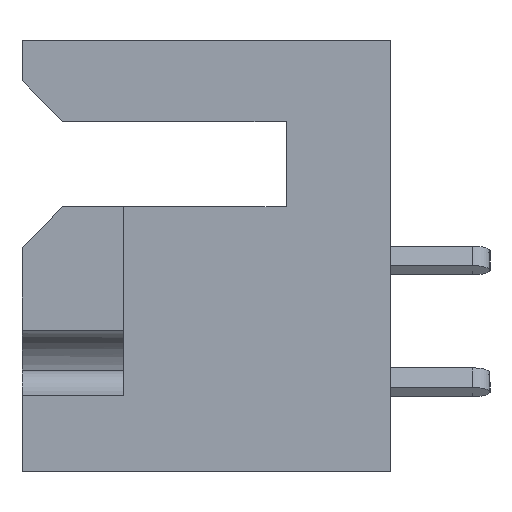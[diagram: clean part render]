
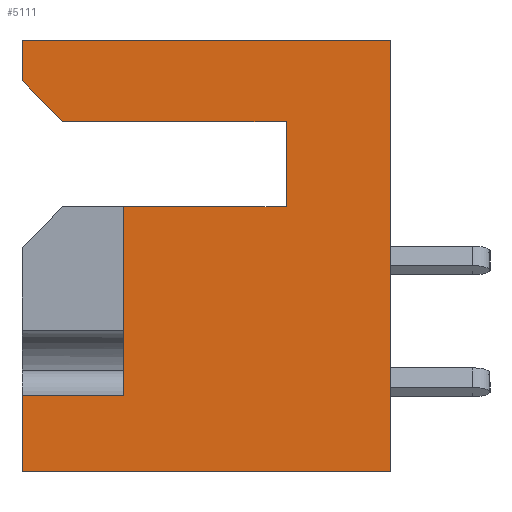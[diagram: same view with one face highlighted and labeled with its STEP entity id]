
A CAD part, left-side view. The second image highlights one B-rep face of the part: STEP entity #5111.
In plain terms, the highlighted planar face has unit normal (-1, 0, 0).
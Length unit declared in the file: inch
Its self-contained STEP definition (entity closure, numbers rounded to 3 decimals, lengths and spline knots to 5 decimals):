
#319 = VECTOR ( 'NONE', #18243, 39.37008 ) ;
#774 = ORIENTED_EDGE ( 'NONE', *, *, #8743, .T. ) ;
#1271 = CARTESIAN_POINT ( 'NONE',  ( 0., 0.453, 0. ) ) ;
#1697 = AXIS2_PLACEMENT_3D ( 'NONE', #1271, #28110, #20865 ) ;
#1863 = CARTESIAN_POINT ( 'NONE',  ( 0., 0.128, -0.1 ) ) ;
#2081 = CARTESIAN_POINT ( 'NONE',  ( 0., 0.453, -0.531 ) ) ;
#2259 = VERTEX_POINT ( 'NONE', #21625 ) ;
#2422 = CARTESIAN_POINT ( 'NONE',  ( 0., 0.328, -0.205 ) ) ;
#3180 = ORIENTED_EDGE ( 'NONE', *, *, #5349, .T. ) ;
#3526 = CARTESIAN_POINT ( 'NONE',  ( 0., 0.403, -0.1 ) ) ;
#3631 = VERTEX_POINT ( 'NONE', #2422 ) ;
#3748 = ORIENTED_EDGE ( 'NONE', *, *, #29592, .T. ) ;
#4726 = LINE ( 'NONE', #18742, #27573 ) ;
#4788 = DIRECTION ( 'NONE',  ( 0., -1., 0. ) ) ;
#5111 = ADVANCED_FACE ( 'NONE', ( #18827 ), #25651, .F. ) ;
#5130 = EDGE_CURVE ( 'NONE', #6974, #15031, #21159, .T. ) ;
#5163 = VERTEX_POINT ( 'NONE', #20975 ) ;
#5301 = VERTEX_POINT ( 'NONE', #15637 ) ;
#5349 = EDGE_CURVE ( 'NONE', #24979, #2259, #16015, .T. ) ;
#6956 = CARTESIAN_POINT ( 'NONE',  ( 0., 0.328, -0.205 ) ) ;
#6965 = LINE ( 'NONE', #28628, #15486 ) ;
#6974 = VERTEX_POINT ( 'NONE', #13891 ) ;
#8162 = EDGE_LOOP ( 'NONE', ( #16756, #13277, #3180, #21647, #12070, #14055, #3748, #29964, #10907, #774, #22965 ) ) ;
#8743 = EDGE_CURVE ( 'NONE', #31337, #3631, #24182, .T. ) ;
#9097 = LINE ( 'NONE', #16215, #21445 ) ;
#9477 = DIRECTION ( 'NONE',  ( 0., 0., 1. ) ) ;
#9629 = LINE ( 'NONE', #1863, #21996 ) ;
#10077 = LINE ( 'NONE', #15993, #319 ) ;
#10907 = ORIENTED_EDGE ( 'NONE', *, *, #18606, .F. ) ;
#11941 = DIRECTION ( 'NONE',  ( 0., 1., 0. ) ) ;
#11972 = EDGE_CURVE ( 'NONE', #15031, #5301, #9097, .T. ) ;
#12070 = ORIENTED_EDGE ( 'NONE', *, *, #11972, .F. ) ;
#13277 = ORIENTED_EDGE ( 'NONE', *, *, #14913, .F. ) ;
#13324 = CARTESIAN_POINT ( 'NONE',  ( 0., 0.453, 0. ) ) ;
#13398 = VERTEX_POINT ( 'NONE', #17681 ) ;
#13711 = EDGE_CURVE ( 'NONE', #5163, #18900, #4726, .T. ) ;
#13891 = CARTESIAN_POINT ( 'NONE',  ( 0., 0.453, -0.05 ) ) ;
#14055 = ORIENTED_EDGE ( 'NONE', *, *, #5130, .F. ) ;
#14740 = VERTEX_POINT ( 'NONE', #3526 ) ;
#14898 = LINE ( 'NONE', #24239, #19511 ) ;
#14913 = EDGE_CURVE ( 'NONE', #24979, #18900, #6965, .T. ) ;
#15031 = VERTEX_POINT ( 'NONE', #29075 ) ;
#15486 = VECTOR ( 'NONE', #28841, 39.37008 ) ;
#15637 = CARTESIAN_POINT ( 'NONE',  ( 0., 0., 0. ) ) ;
#15993 = CARTESIAN_POINT ( 'NONE',  ( 0., 0.128, -0.1 ) ) ;
#16015 = LINE ( 'NONE', #2081, #25332 ) ;
#16215 = CARTESIAN_POINT ( 'NONE',  ( 0., 0.453, 0. ) ) ;
#16589 = EDGE_CURVE ( 'NONE', #5163, #3631, #20771, .T. ) ;
#16756 = ORIENTED_EDGE ( 'NONE', *, *, #13711, .T. ) ;
#16796 = DIRECTION ( 'NONE',  ( 0., 1., 0. ) ) ;
#17681 = CARTESIAN_POINT ( 'NONE',  ( 0., 0.128, -0.1 ) ) ;
#18243 = DIRECTION ( 'NONE',  ( 0., 0., 1. ) ) ;
#18606 = EDGE_CURVE ( 'NONE', #31337, #13398, #10077, .T. ) ;
#18742 = CARTESIAN_POINT ( 'NONE',  ( 0., 0.328, -0.437 ) ) ;
#18827 = FACE_OUTER_BOUND ( 'NONE', #8162, .T. ) ;
#18900 = VERTEX_POINT ( 'NONE', #29178 ) ;
#19511 = VECTOR ( 'NONE', #20074, 39.37008 ) ;
#19580 = EDGE_CURVE ( 'NONE', #13398, #14740, #9629, .T. ) ;
#20035 = CARTESIAN_POINT ( 'NONE',  ( 0., 0.128, -0.205 ) ) ;
#20074 = DIRECTION ( 'NONE',  ( 0., 0., 1. ) ) ;
#20771 = LINE ( 'NONE', #6956, #26961 ) ;
#20865 = DIRECTION ( 'NONE',  ( 0., 0., -1. ) ) ;
#20975 = CARTESIAN_POINT ( 'NONE',  ( 0., 0.328, -0.437 ) ) ;
#21083 = DIRECTION ( 'NONE',  ( 0., 0., 1. ) ) ;
#21159 = LINE ( 'NONE', #13324, #26978 ) ;
#21445 = VECTOR ( 'NONE', #28319, 39.37008 ) ;
#21625 = CARTESIAN_POINT ( 'NONE',  ( 0., 0., -0.531 ) ) ;
#21647 = ORIENTED_EDGE ( 'NONE', *, *, #28227, .T. ) ;
#21764 = VECTOR ( 'NONE', #29117, 39.37008 ) ;
#21996 = VECTOR ( 'NONE', #11941, 39.37008 ) ;
#22058 = CARTESIAN_POINT ( 'NONE',  ( 0., 0.453, -0.531 ) ) ;
#22093 = CARTESIAN_POINT ( 'NONE',  ( 0., 0.403, -0.1 ) ) ;
#22965 = ORIENTED_EDGE ( 'NONE', *, *, #16589, .F. ) ;
#24182 = LINE ( 'NONE', #29368, #26070 ) ;
#24239 = CARTESIAN_POINT ( 'NONE',  ( 0., 0., 0. ) ) ;
#24979 = VERTEX_POINT ( 'NONE', #22058 ) ;
#25332 = VECTOR ( 'NONE', #4788, 39.37008 ) ;
#25651 = PLANE ( 'NONE',  #1697 ) ;
#26070 = VECTOR ( 'NONE', #26564, 39.37008 ) ;
#26564 = DIRECTION ( 'NONE',  ( 0., 1., 0. ) ) ;
#26961 = VECTOR ( 'NONE', #9477, 39.37008 ) ;
#26978 = VECTOR ( 'NONE', #21083, 39.37008 ) ;
#27573 = VECTOR ( 'NONE', #16796, 39.37008 ) ;
#28110 = DIRECTION ( 'NONE',  ( 1., 0., 0. ) ) ;
#28227 = EDGE_CURVE ( 'NONE', #2259, #5301, #14898, .T. ) ;
#28319 = DIRECTION ( 'NONE',  ( 0., -1., 0. ) ) ;
#28628 = CARTESIAN_POINT ( 'NONE',  ( 0., 0.453, 0. ) ) ;
#28841 = DIRECTION ( 'NONE',  ( 0., 0., 1. ) ) ;
#29075 = CARTESIAN_POINT ( 'NONE',  ( 0., 0.453, 0. ) ) ;
#29117 = DIRECTION ( 'NONE',  ( 0., -0.707, -0.707 ) ) ;
#29178 = CARTESIAN_POINT ( 'NONE',  ( 0., 0.453, -0.437 ) ) ;
#29368 = CARTESIAN_POINT ( 'NONE',  ( 0., 0.128, -0.205 ) ) ;
#29592 = EDGE_CURVE ( 'NONE', #6974, #14740, #31452, .T. ) ;
#29964 = ORIENTED_EDGE ( 'NONE', *, *, #19580, .F. ) ;
#31337 = VERTEX_POINT ( 'NONE', #20035 ) ;
#31452 = LINE ( 'NONE', #22093, #21764 ) ;
